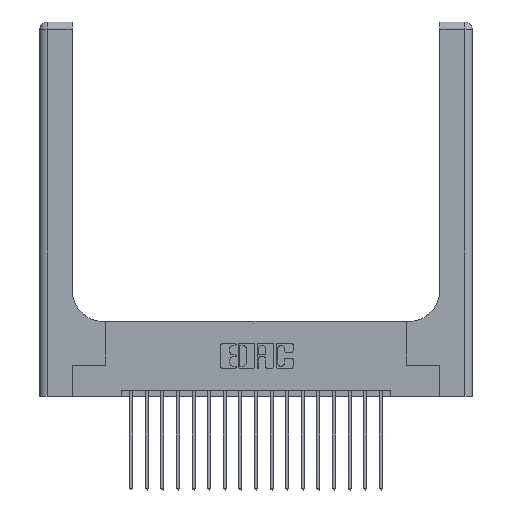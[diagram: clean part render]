
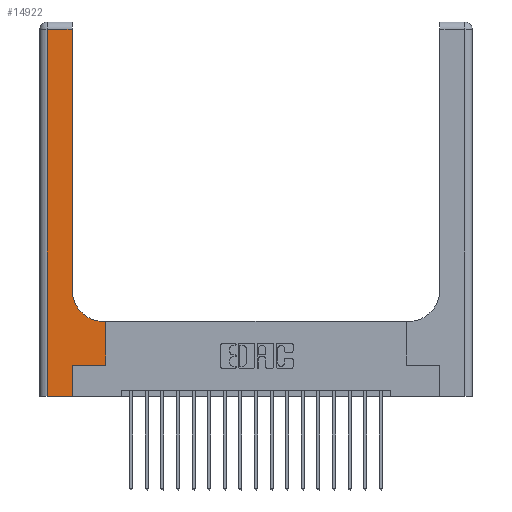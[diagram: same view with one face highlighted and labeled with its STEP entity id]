
A CAD part, top view. The second image highlights one B-rep face of the part: STEP entity #14922.
In plain terms, the highlighted planar face has unit normal (0, 0, 1).
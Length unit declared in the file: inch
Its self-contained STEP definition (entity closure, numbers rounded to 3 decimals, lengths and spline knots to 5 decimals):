
#83 = LINE ( 'NONE', #12770, #7245 ) ;
#141 = EDGE_CURVE ( 'NONE', #18512, #13171, #18185, .T. ) ;
#251 = ORIENTED_EDGE ( 'NONE', *, *, #141, .T. ) ;
#574 = LINE ( 'NONE', #1745, #14624 ) ;
#715 = VERTEX_POINT ( 'NONE', #3913 ) ;
#781 = VECTOR ( 'NONE', #4261, 39.37008 ) ;
#1189 = EDGE_CURVE ( 'NONE', #715, #19458, #2259, .T. ) ;
#1290 = CARTESIAN_POINT ( 'NONE',  ( 0.06, 3., 0.37 ) ) ;
#1335 = CARTESIAN_POINT ( 'NONE',  ( 0.06, 0., 0.37 ) ) ;
#1679 = DIRECTION ( 'NONE',  ( -1., 0., 0. ) ) ;
#1745 = CARTESIAN_POINT ( 'NONE',  ( 0.26, 0.6, 0.37 ) ) ;
#2006 = ORIENTED_EDGE ( 'NONE', *, *, #1189, .T. ) ;
#2259 = LINE ( 'NONE', #2394, #17448 ) ;
#2394 = CARTESIAN_POINT ( 'NONE',  ( 0.265, 0., 0.37 ) ) ;
#2570 = LINE ( 'NONE', #18141, #9475 ) ;
#2894 = VERTEX_POINT ( 'NONE', #9441 ) ;
#2919 = LINE ( 'NONE', #18778, #13585 ) ;
#3053 = LINE ( 'NONE', #16768, #17053 ) ;
#3350 = DIRECTION ( 'NONE',  ( 0., 1., 0. ) ) ;
#3536 = VECTOR ( 'NONE', #12448, 39.37008 ) ;
#3913 = CARTESIAN_POINT ( 'NONE',  ( 0.265, 0., 0.37 ) ) ;
#4043 = DIRECTION ( 'NONE',  ( 1., 0., 0. ) ) ;
#4261 = DIRECTION ( 'NONE',  ( 0., -1., 0. ) ) ;
#5487 = EDGE_LOOP ( 'NONE', ( #11979, #7904, #13101, #8787, #2006, #6291, #9258, #5993, #251 ) ) ;
#5993 = ORIENTED_EDGE ( 'NONE', *, *, #14415, .T. ) ;
#6291 = ORIENTED_EDGE ( 'NONE', *, *, #19347, .T. ) ;
#6754 = EDGE_CURVE ( 'NONE', #2894, #7229, #83, .T. ) ;
#7148 = AXIS2_PLACEMENT_3D ( 'NONE', #16140, #8465, #17784 ) ;
#7229 = VERTEX_POINT ( 'NONE', #9816 ) ;
#7245 = VECTOR ( 'NONE', #11115, 39.37008 ) ;
#7833 = DIRECTION ( 'NONE',  ( 0., 1., 0. ) ) ;
#7882 = AXIS2_PLACEMENT_3D ( 'NONE', #11284, #18998, #4043 ) ;
#7904 = ORIENTED_EDGE ( 'NONE', *, *, #6754, .T. ) ;
#8030 = EDGE_CURVE ( 'NONE', #15275, #8407, #2919, .T. ) ;
#8037 = CARTESIAN_POINT ( 'NONE',  ( 0., 0., 0.37 ) ) ;
#8407 = VERTEX_POINT ( 'NONE', #16464 ) ;
#8465 = DIRECTION ( 'NONE',  ( 0., 0., -1. ) ) ;
#8612 = DIRECTION ( 'NONE',  ( 0., 1., 0. ) ) ;
#8787 = ORIENTED_EDGE ( 'NONE', *, *, #11759, .T. ) ;
#9258 = ORIENTED_EDGE ( 'NONE', *, *, #8030, .T. ) ;
#9441 = CARTESIAN_POINT ( 'NONE',  ( 0.26, 2.94, 0.37 ) ) ;
#9475 = VECTOR ( 'NONE', #16667, 39.37008 ) ;
#9583 = CARTESIAN_POINT ( 'NONE',  ( 0.265, 0.25, 0.37 ) ) ;
#9816 = CARTESIAN_POINT ( 'NONE',  ( 0.06, 2.94, 0.37 ) ) ;
#10567 = FACE_OUTER_BOUND ( 'NONE', #5487, .T. ) ;
#11115 = DIRECTION ( 'NONE',  ( -1., 0., 0. ) ) ;
#11284 = CARTESIAN_POINT ( 'NONE',  ( 0.51, 0.85, 0.37 ) ) ;
#11759 = EDGE_CURVE ( 'NONE', #18948, #715, #14691, .T. ) ;
#11979 = ORIENTED_EDGE ( 'NONE', *, *, #12711, .T. ) ;
#12448 = DIRECTION ( 'NONE',  ( 1., 0., 0. ) ) ;
#12711 = EDGE_CURVE ( 'NONE', #13171, #2894, #3053, .T. ) ;
#12770 = CARTESIAN_POINT ( 'NONE',  ( 0., 2.94, 0.37 ) ) ;
#13101 = ORIENTED_EDGE ( 'NONE', *, *, #15040, .T. ) ;
#13171 = VERTEX_POINT ( 'NONE', #16121 ) ;
#13585 = VECTOR ( 'NONE', #3350, 39.37008 ) ;
#13995 = CARTESIAN_POINT ( 'NONE',  ( 0.51, 0.6, 0.37 ) ) ;
#14415 = EDGE_CURVE ( 'NONE', #8407, #18512, #574, .T. ) ;
#14426 = CARTESIAN_POINT ( 'NONE',  ( 0.528, 0.25, 0.37 ) ) ;
#14624 = VECTOR ( 'NONE', #1679, 39.37008 ) ;
#14691 = LINE ( 'NONE', #8037, #3536 ) ;
#14744 = PLANE ( 'NONE',  #7148 ) ;
#14922 = ADVANCED_FACE ( 'NONE', ( #10567 ), #14744, .F. ) ;
#15040 = EDGE_CURVE ( 'NONE', #7229, #18948, #16008, .T. ) ;
#15275 = VERTEX_POINT ( 'NONE', #14426 ) ;
#16008 = LINE ( 'NONE', #1290, #781 ) ;
#16121 = CARTESIAN_POINT ( 'NONE',  ( 0.26, 0.85, 0.37 ) ) ;
#16140 = CARTESIAN_POINT ( 'NONE',  ( 0., 3., 0.37 ) ) ;
#16464 = CARTESIAN_POINT ( 'NONE',  ( 0.528, 0.6, 0.37 ) ) ;
#16667 = DIRECTION ( 'NONE',  ( 1., 0., 0. ) ) ;
#16768 = CARTESIAN_POINT ( 'NONE',  ( 0.26, 3., 0.37 ) ) ;
#17053 = VECTOR ( 'NONE', #7833, 39.37008 ) ;
#17448 = VECTOR ( 'NONE', #8612, 39.37008 ) ;
#17784 = DIRECTION ( 'NONE',  ( -1., 0., 0. ) ) ;
#18141 = CARTESIAN_POINT ( 'NONE',  ( 0.265, 0.25, 0.37 ) ) ;
#18185 = CIRCLE ( 'NONE', #7882, 0.25 ) ;
#18512 = VERTEX_POINT ( 'NONE', #13995 ) ;
#18778 = CARTESIAN_POINT ( 'NONE',  ( 0.528, 0.25, 0.37 ) ) ;
#18948 = VERTEX_POINT ( 'NONE', #1335 ) ;
#18998 = DIRECTION ( 'NONE',  ( 0., 0., -1. ) ) ;
#19347 = EDGE_CURVE ( 'NONE', #19458, #15275, #2570, .T. ) ;
#19458 = VERTEX_POINT ( 'NONE', #9583 ) ;
